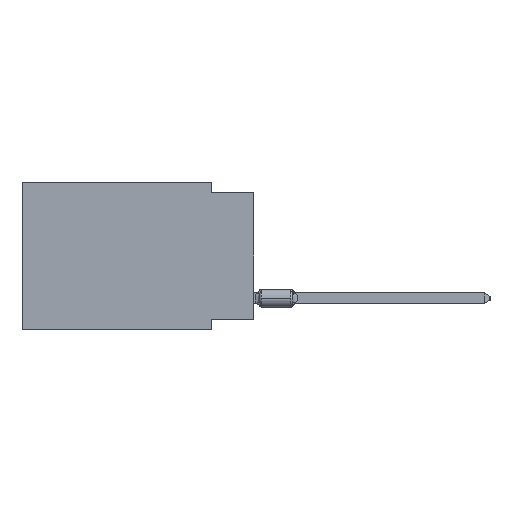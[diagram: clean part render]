
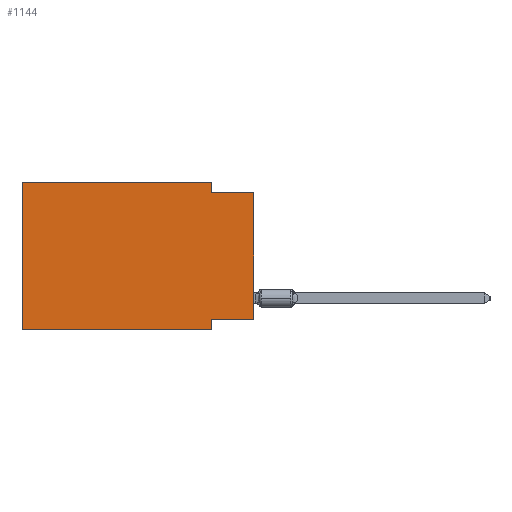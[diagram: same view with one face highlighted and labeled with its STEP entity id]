
A CAD part, left-side view. The second image highlights one B-rep face of the part: STEP entity #1144.
In plain terms, the highlighted planar face has unit normal (-1, 0, 0).
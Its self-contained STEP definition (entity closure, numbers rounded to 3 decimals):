
#219 = EDGE_CURVE ( 'NONE', #26822, #44275, #29928, .T. ) ;
#702 = VECTOR ( 'NONE', #44368, 1000. ) ;
#802 = LINE ( 'NONE', #48373, #44497 ) ;
#1144 = ADVANCED_FACE ( 'NONE', ( #31306 ), #7525, .F. ) ;
#3077 = CARTESIAN_POINT ( 'NONE',  ( 0., 2.54, -8.255 ) ) ;
#4219 = CARTESIAN_POINT ( 'NONE',  ( 0., 13.97, 0. ) ) ;
#4678 = CARTESIAN_POINT ( 'NONE',  ( 0., 0., -0.635 ) ) ;
#4999 = ORIENTED_EDGE ( 'NONE', *, *, #18610, .F. ) ;
#5600 = VERTEX_POINT ( 'NONE', #23230 ) ;
#6106 = DIRECTION ( 'NONE',  ( 0., 0., -1. ) ) ;
#6364 = VECTOR ( 'NONE', #6106, 1000. ) ;
#6453 = CARTESIAN_POINT ( 'NONE',  ( 0., 2.54, -0.635 ) ) ;
#6626 = EDGE_LOOP ( 'NONE', ( #19592, #4999, #7188, #13623, #49806, #29574, #16656, #45918 ) ) ;
#7188 = ORIENTED_EDGE ( 'NONE', *, *, #50111, .F. ) ;
#7525 = PLANE ( 'NONE',  #31792 ) ;
#8760 = VECTOR ( 'NONE', #16814, 1000. ) ;
#11660 = LINE ( 'NONE', #15027, #17133 ) ;
#12019 = VERTEX_POINT ( 'NONE', #6453 ) ;
#13623 = ORIENTED_EDGE ( 'NONE', *, *, #36475, .F. ) ;
#14416 = CARTESIAN_POINT ( 'NONE',  ( 0., 0., 0. ) ) ;
#15027 = CARTESIAN_POINT ( 'NONE',  ( 0., 0., -8.255 ) ) ;
#15456 = CARTESIAN_POINT ( 'NONE',  ( 0., 2.54, -8.89 ) ) ;
#16574 = DIRECTION ( 'NONE',  ( 0., -1., 0. ) ) ;
#16656 = ORIENTED_EDGE ( 'NONE', *, *, #49036, .F. ) ;
#16814 = DIRECTION ( 'NONE',  ( 0., -1., 0. ) ) ;
#16934 = LINE ( 'NONE', #28573, #702 ) ;
#17133 = VECTOR ( 'NONE', #23052, 1000. ) ;
#17735 = LINE ( 'NONE', #22652, #6364 ) ;
#18610 = EDGE_CURVE ( 'NONE', #12019, #44275, #25345, .T. ) ;
#19592 = ORIENTED_EDGE ( 'NONE', *, *, #219, .T. ) ;
#19740 = LINE ( 'NONE', #4219, #49334 ) ;
#19910 = DIRECTION ( 'NONE',  ( 1., 0., 0. ) ) ;
#22004 = CARTESIAN_POINT ( 'NONE',  ( 0., 0., -8.255 ) ) ;
#22652 = CARTESIAN_POINT ( 'NONE',  ( 0., 2.54, 0. ) ) ;
#23052 = DIRECTION ( 'NONE',  ( 0., 1., 0. ) ) ;
#23230 = CARTESIAN_POINT ( 'NONE',  ( 0., 13.97, -8.89 ) ) ;
#25345 = LINE ( 'NONE', #4678, #8760 ) ;
#25805 = DIRECTION ( 'NONE',  ( 0., 0., 1. ) ) ;
#26822 = VERTEX_POINT ( 'NONE', #22004 ) ;
#28573 = CARTESIAN_POINT ( 'NONE',  ( 0., 13.97, 0. ) ) ;
#29574 = ORIENTED_EDGE ( 'NONE', *, *, #45455, .T. ) ;
#29898 = CARTESIAN_POINT ( 'NONE',  ( 0., 2.54, -8.89 ) ) ;
#29928 = LINE ( 'NONE', #14416, #32570 ) ;
#31306 = FACE_OUTER_BOUND ( 'NONE', #6626, .T. ) ;
#31381 = VERTEX_POINT ( 'NONE', #44272 ) ;
#31792 = AXIS2_PLACEMENT_3D ( 'NONE', #43458, #19910, #39583 ) ;
#32570 = VECTOR ( 'NONE', #25805, 1000. ) ;
#32782 = EDGE_CURVE ( 'NONE', #26822, #33152, #11660, .T. ) ;
#33152 = VERTEX_POINT ( 'NONE', #3077 ) ;
#33245 = CARTESIAN_POINT ( 'NONE',  ( 0., 13.97, 0. ) ) ;
#36475 = EDGE_CURVE ( 'NONE', #49996, #31381, #16934, .T. ) ;
#39583 = DIRECTION ( 'NONE',  ( 0., 0., -1. ) ) ;
#41302 = LINE ( 'NONE', #29898, #49211 ) ;
#41369 = CARTESIAN_POINT ( 'NONE',  ( 0., 0., -0.635 ) ) ;
#41548 = DIRECTION ( 'NONE',  ( 0., 0., -1. ) ) ;
#42039 = EDGE_CURVE ( 'NONE', #5600, #49996, #19740, .T. ) ;
#43272 = DIRECTION ( 'NONE',  ( 0., 0., 1. ) ) ;
#43458 = CARTESIAN_POINT ( 'NONE',  ( 0., 13.97, 0. ) ) ;
#44272 = CARTESIAN_POINT ( 'NONE',  ( 0., 2.54, 0. ) ) ;
#44275 = VERTEX_POINT ( 'NONE', #41369 ) ;
#44368 = DIRECTION ( 'NONE',  ( 0., -1., 0. ) ) ;
#44497 = VECTOR ( 'NONE', #16574, 1000. ) ;
#45455 = EDGE_CURVE ( 'NONE', #5600, #49946, #802, .T. ) ;
#45918 = ORIENTED_EDGE ( 'NONE', *, *, #32782, .F. ) ;
#48373 = CARTESIAN_POINT ( 'NONE',  ( 0., 13.97, -8.89 ) ) ;
#49036 = EDGE_CURVE ( 'NONE', #33152, #49946, #41302, .T. ) ;
#49211 = VECTOR ( 'NONE', #41548, 1000. ) ;
#49334 = VECTOR ( 'NONE', #43272, 1000. ) ;
#49806 = ORIENTED_EDGE ( 'NONE', *, *, #42039, .F. ) ;
#49946 = VERTEX_POINT ( 'NONE', #15456 ) ;
#49996 = VERTEX_POINT ( 'NONE', #33245 ) ;
#50111 = EDGE_CURVE ( 'NONE', #31381, #12019, #17735, .T. ) ;
